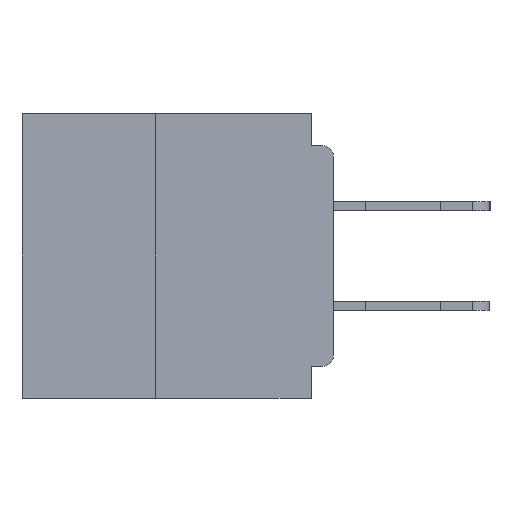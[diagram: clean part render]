
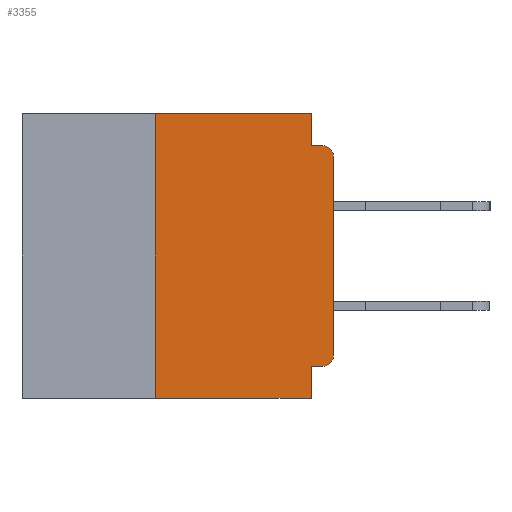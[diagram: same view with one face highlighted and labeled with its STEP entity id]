
A CAD part, left-side view. The second image highlights one B-rep face of the part: STEP entity #3355.
In plain terms, the highlighted planar face has unit normal (-1, 0, 0).
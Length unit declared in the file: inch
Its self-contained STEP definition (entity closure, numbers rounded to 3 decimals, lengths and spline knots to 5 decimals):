
#197 = CARTESIAN_POINT ( 'NONE',  ( 0., 0.25, -0.4 ) ) ;
#301 = DIRECTION ( 'NONE',  ( 0., 0., -1. ) ) ;
#959 = VERTEX_POINT ( 'NONE', #36987 ) ;
#1224 = DIRECTION ( 'NONE',  ( 0., -1., 0. ) ) ;
#1843 = CARTESIAN_POINT ( 'NONE',  ( 0., 0.437, 0. ) ) ;
#1917 = EDGE_CURVE ( 'NONE', #14443, #14397, #38593, .T. ) ;
#2560 = CARTESIAN_POINT ( 'NONE',  ( 0., 0.015, -0.34 ) ) ;
#2602 = ORIENTED_EDGE ( 'NONE', *, *, #45628, .T. ) ;
#2874 = ORIENTED_EDGE ( 'NONE', *, *, #29742, .F. ) ;
#3355 = ADVANCED_FACE ( 'NONE', ( #43043 ), #10981, .F. ) ;
#3790 = CARTESIAN_POINT ( 'NONE',  ( 0., 0.031, -0.355 ) ) ;
#3805 = CARTESIAN_POINT ( 'NONE',  ( 0., 0.25, 0. ) ) ;
#4717 = LINE ( 'NONE', #35973, #41922 ) ;
#5120 = CARTESIAN_POINT ( 'NONE',  ( 0., 0.015, -0.355 ) ) ;
#5400 = DIRECTION ( 'NONE',  ( 0., -1., 0. ) ) ;
#5479 = ORIENTED_EDGE ( 'NONE', *, *, #24856, .T. ) ;
#6107 = ORIENTED_EDGE ( 'NONE', *, *, #8562, .F. ) ;
#6119 = DIRECTION ( 'NONE',  ( 0., 0., -1. ) ) ;
#6483 = LINE ( 'NONE', #8382, #14976 ) ;
#6750 = ORIENTED_EDGE ( 'NONE', *, *, #19706, .T. ) ;
#6773 = EDGE_LOOP ( 'NONE', ( #6750, #5479, #2874, #19908, #6107, #23314, #22442, #25121, #25886, #2602 ) ) ;
#7029 = LINE ( 'NONE', #1843, #25015 ) ;
#7556 = VERTEX_POINT ( 'NONE', #42048 ) ;
#8350 = DIRECTION ( 'NONE',  ( -1., 0., 0. ) ) ;
#8382 = CARTESIAN_POINT ( 'NONE',  ( 0., 0.031, -0.4 ) ) ;
#8562 = EDGE_CURVE ( 'NONE', #14397, #9203, #7029, .T. ) ;
#9203 = VERTEX_POINT ( 'NONE', #11348 ) ;
#10981 = PLANE ( 'NONE',  #38512 ) ;
#11348 = CARTESIAN_POINT ( 'NONE',  ( 0., 0.031, 0. ) ) ;
#13224 = VECTOR ( 'NONE', #1224, 39.37008 ) ;
#13753 = DIRECTION ( 'NONE',  ( 0., 0., 1. ) ) ;
#13942 = EDGE_CURVE ( 'NONE', #26697, #16184, #6483, .T. ) ;
#14397 = VERTEX_POINT ( 'NONE', #3805 ) ;
#14443 = VERTEX_POINT ( 'NONE', #197 ) ;
#14924 = CARTESIAN_POINT ( 'NONE',  ( 0., 0.015, -0.045 ) ) ;
#14976 = VECTOR ( 'NONE', #33622, 39.37008 ) ;
#16184 = VERTEX_POINT ( 'NONE', #21725 ) ;
#16960 = EDGE_CURVE ( 'NONE', #26061, #26697, #45738, .T. ) ;
#17010 = VECTOR ( 'NONE', #23072, 39.37008 ) ;
#18012 = DIRECTION ( 'NONE',  ( 0., 0., -1. ) ) ;
#18261 = CARTESIAN_POINT ( 'NONE',  ( 0., 0.437, -0.4 ) ) ;
#19404 = VECTOR ( 'NONE', #35895, 39.37008 ) ;
#19478 = CARTESIAN_POINT ( 'NONE',  ( 0., 0., -0.355 ) ) ;
#19706 = EDGE_CURVE ( 'NONE', #7556, #25510, #30875, .T. ) ;
#19908 = ORIENTED_EDGE ( 'NONE', *, *, #30156, .F. ) ;
#20120 = VECTOR ( 'NONE', #13753, 39.37008 ) ;
#21725 = CARTESIAN_POINT ( 'NONE',  ( 0., 0.031, -0.4 ) ) ;
#21810 = DIRECTION ( 'NONE',  ( 1., 0., 0. ) ) ;
#22442 = ORIENTED_EDGE ( 'NONE', *, *, #44041, .T. ) ;
#23072 = DIRECTION ( 'NONE',  ( 0., 1., 0. ) ) ;
#23314 = ORIENTED_EDGE ( 'NONE', *, *, #1917, .F. ) ;
#24856 = EDGE_CURVE ( 'NONE', #25510, #31440, #40625, .T. ) ;
#25015 = VECTOR ( 'NONE', #5400, 39.37008 ) ;
#25121 = ORIENTED_EDGE ( 'NONE', *, *, #13942, .F. ) ;
#25510 = VERTEX_POINT ( 'NONE', #33542 ) ;
#25886 = ORIENTED_EDGE ( 'NONE', *, *, #16960, .F. ) ;
#26061 = VERTEX_POINT ( 'NONE', #5120 ) ;
#26697 = VERTEX_POINT ( 'NONE', #3790 ) ;
#27661 = DIRECTION ( 'NONE',  ( -1., 0., 0. ) ) ;
#29083 = DIRECTION ( 'NONE',  ( 0., -1., 0. ) ) ;
#29742 = EDGE_CURVE ( 'NONE', #959, #31440, #41965, .T. ) ;
#29942 = CARTESIAN_POINT ( 'NONE',  ( 0., 0.015, -0.06 ) ) ;
#30156 = EDGE_CURVE ( 'NONE', #9203, #959, #4717, .T. ) ;
#30875 = LINE ( 'NONE', #35320, #20120 ) ;
#31440 = VERTEX_POINT ( 'NONE', #14924 ) ;
#33512 = CARTESIAN_POINT ( 'NONE',  ( 0., 0., -0.045 ) ) ;
#33542 = CARTESIAN_POINT ( 'NONE',  ( 0., 0., -0.06 ) ) ;
#33595 = DIRECTION ( 'NONE',  ( 0., 0., -1. ) ) ;
#33622 = DIRECTION ( 'NONE',  ( 0., 0., -1. ) ) ;
#35320 = CARTESIAN_POINT ( 'NONE',  ( 0., 0., 0. ) ) ;
#35895 = DIRECTION ( 'NONE',  ( 0., 0., 1. ) ) ;
#35940 = CARTESIAN_POINT ( 'NONE',  ( 0., 0.25, -0.4 ) ) ;
#35973 = CARTESIAN_POINT ( 'NONE',  ( 0., 0.031, 0. ) ) ;
#36987 = CARTESIAN_POINT ( 'NONE',  ( 0., 0.031, -0.045 ) ) ;
#38430 = VECTOR ( 'NONE', #29083, 39.37008 ) ;
#38512 = AXIS2_PLACEMENT_3D ( 'NONE', #43278, #21810, #301 ) ;
#38593 = LINE ( 'NONE', #35940, #19404 ) ;
#39850 = AXIS2_PLACEMENT_3D ( 'NONE', #2560, #27661, #6119 ) ;
#40625 = CIRCLE ( 'NONE', #46454, 0.015 ) ;
#40710 = LINE ( 'NONE', #18261, #38430 ) ;
#41922 = VECTOR ( 'NONE', #18012, 39.37008 ) ;
#41965 = LINE ( 'NONE', #33512, #13224 ) ;
#42048 = CARTESIAN_POINT ( 'NONE',  ( 0., 0., -0.34 ) ) ;
#43043 = FACE_OUTER_BOUND ( 'NONE', #6773, .T. ) ;
#43278 = CARTESIAN_POINT ( 'NONE',  ( 0., 0.437, 0. ) ) ;
#44041 = EDGE_CURVE ( 'NONE', #14443, #16184, #40710, .T. ) ;
#45628 = EDGE_CURVE ( 'NONE', #26061, #7556, #45667, .T. ) ;
#45667 = CIRCLE ( 'NONE', #39850, 0.015 ) ;
#45738 = LINE ( 'NONE', #19478, #17010 ) ;
#46454 = AXIS2_PLACEMENT_3D ( 'NONE', #29942, #8350, #33595 ) ;
